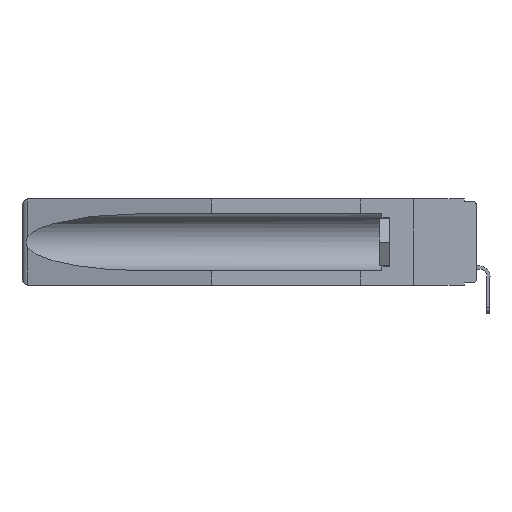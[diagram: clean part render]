
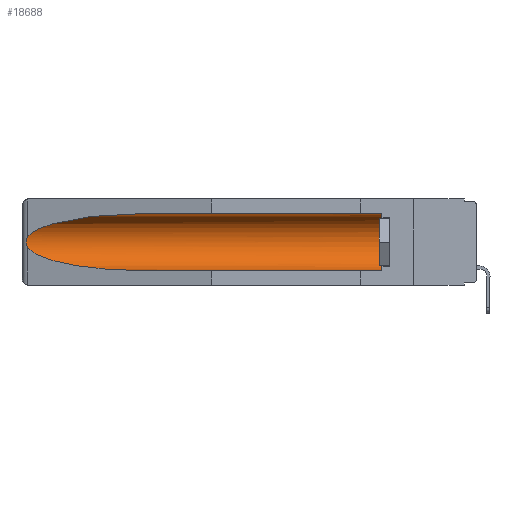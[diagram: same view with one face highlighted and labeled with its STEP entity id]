
A CAD part, left-side view. The second image highlights one B-rep face of the part: STEP entity #18688.
In plain terms, the highlighted cylindrical face has radius 2.857 mm (diameter 5.715 mm), a partial arc.
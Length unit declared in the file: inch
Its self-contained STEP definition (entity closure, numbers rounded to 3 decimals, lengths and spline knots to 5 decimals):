
#214 =( BOUNDED_CURVE ( )  B_SPLINE_CURVE ( 3, ( #3086, #10755, #3312, #23945 ),
 .UNSPECIFIED., .F., .F. ) 
 B_SPLINE_CURVE_WITH_KNOTS ( ( 4, 4 ),
 ( 0.1948, 1.5708 ),
 .UNSPECIFIED. ) 
 CURVE ( )  GEOMETRIC_REPRESENTATION_ITEM ( )  RATIONAL_B_SPLINE_CURVE ( ( 1., 0.848, 0.848, 1. ) ) 
 REPRESENTATION_ITEM ( '' )  );
#909 = CARTESIAN_POINT ( 'NONE',  ( 0.2675, 1.53308, -0.17534 ) ) ;
#1145 = CARTESIAN_POINT ( 'NONE',  ( 0.155, 0.126, -0.1715 ) ) ;
#1150 = CARTESIAN_POINT ( 'NONE',  ( 0.26597, 1.5296, -0.19026 ) ) ;
#1480 = ORIENTED_EDGE ( 'NONE', *, *, #16808, .T. ) ;
#1636 = CARTESIAN_POINT ( 'NONE',  ( 0.155, 1.07973, -0.284 ) ) ;
#1738 = B_SPLINE_CURVE_WITH_KNOTS ( 'NONE', 3,
 ( #10363, #10457, #4682, #23730, #18011, #909, #14199, #2793, #1150, #3044 ),
 .UNSPECIFIED., .F., .F.,
 ( 4, 2, 2, 2, 4 ),
 ( 0., 0.00029, 0.00058, 0.00087, 0.00117 ),
 .UNSPECIFIED. ) ;
#2286 = EDGE_CURVE ( 'NONE', #7174, #4447, #18360, .T. ) ;
#2654 = CARTESIAN_POINT ( 'NONE',  ( 0.155, -0.30754, -0.059 ) ) ;
#2793 = CARTESIAN_POINT ( 'NONE',  ( 0.26655, 1.53094, -0.18657 ) ) ;
#2854 = EDGE_CURVE ( 'NONE', #22755, #12830, #214, .T. ) ;
#3044 = CARTESIAN_POINT ( 'NONE',  ( 0.26537, 1.52718, -0.19328 ) ) ;
#3086 = CARTESIAN_POINT ( 'NONE',  ( 0.26537, 1.52718, -0.19328 ) ) ;
#3312 = CARTESIAN_POINT ( 'NONE',  ( 0.21114, 1.30732, -0.284 ) ) ;
#3334 = CARTESIAN_POINT ( 'NONE',  ( 0.155, -0.30754, -0.284 ) ) ;
#4349 = EDGE_LOOP ( 'NONE', ( #18473, #1480, #19409, #7672, #11660, #10160 ) ) ;
#4447 = VERTEX_POINT ( 'NONE', #12825 ) ;
#4682 = CARTESIAN_POINT ( 'NONE',  ( 0.26654, 1.53092, -0.15636 ) ) ;
#5478 = CARTESIAN_POINT ( 'NONE',  ( 0.155, 0.126, -0.284 ) ) ;
#6430 = DIRECTION ( 'NONE',  ( 0., 1., 0. ) ) ;
#6952 = DIRECTION ( 'NONE',  ( 0., 1., 0. ) ) ;
#7174 = VERTEX_POINT ( 'NONE', #5478 ) ;
#7672 = ORIENTED_EDGE ( 'NONE', *, *, #9293, .F. ) ;
#7790 = VECTOR ( 'NONE', #6430, 39.37008 ) ;
#8319 = CARTESIAN_POINT ( 'NONE',  ( 0.26537, 1.52718, -0.14972 ) ) ;
#8668 = DIRECTION ( 'NONE',  ( 0., 0., 1. ) ) ;
#9293 = EDGE_CURVE ( 'NONE', #7174, #12830, #16475, .T. ) ;
#10160 = ORIENTED_EDGE ( 'NONE', *, *, #16293, .T. ) ;
#10363 = CARTESIAN_POINT ( 'NONE',  ( 0.26537, 1.52718, -0.14972 ) ) ;
#10380 = VERTEX_POINT ( 'NONE', #24231 ) ;
#10457 = CARTESIAN_POINT ( 'NONE',  ( 0.26597, 1.52961, -0.15275 ) ) ;
#10755 = CARTESIAN_POINT ( 'NONE',  ( 0.25451, 1.48313, -0.24835 ) ) ;
#11124 = LINE ( 'NONE', #2654, #7790 ) ;
#11408 = VECTOR ( 'NONE', #16687, 39.37008 ) ;
#11660 = ORIENTED_EDGE ( 'NONE', *, *, #2286, .T. ) ;
#11787 = FACE_OUTER_BOUND ( 'NONE', #4349, .T. ) ;
#12029 = CARTESIAN_POINT ( 'NONE',  ( 0.21114, 1.30732, -0.059 ) ) ;
#12825 = CARTESIAN_POINT ( 'NONE',  ( 0.155, 0.126, -0.059 ) ) ;
#12830 = VERTEX_POINT ( 'NONE', #1636 ) ;
#14199 = CARTESIAN_POINT ( 'NONE',  ( 0.2673, 1.53269, -0.17917 ) ) ;
#15849 = CARTESIAN_POINT ( 'NONE',  ( 0.25451, 1.48313, -0.09465 ) ) ;
#16293 = EDGE_CURVE ( 'NONE', #4447, #10380, #11124, .T. ) ;
#16475 = LINE ( 'NONE', #3334, #11408 ) ;
#16501 = CARTESIAN_POINT ( 'NONE',  ( 0.155, -0.30754, -0.1715 ) ) ;
#16566 = CYLINDRICAL_SURFACE ( 'NONE', #23483, 0.1125 ) ;
#16687 = DIRECTION ( 'NONE',  ( 0., 1., 0. ) ) ;
#16808 = EDGE_CURVE ( 'NONE', #18762, #22755, #1738, .T. ) ;
#17666 = CARTESIAN_POINT ( 'NONE',  ( 0.155, 1.07973, -0.059 ) ) ;
#18011 = CARTESIAN_POINT ( 'NONE',  ( 0.2675, 1.53308, -0.16763 ) ) ;
#18360 = CIRCLE ( 'NONE', #19079, 0.1125 ) ;
#18473 = ORIENTED_EDGE ( 'NONE', *, *, #21146, .T. ) ;
#18688 = ADVANCED_FACE ( 'NONE', ( #11787 ), #16566, .F. ) ;
#18762 = VERTEX_POINT ( 'NONE', #21893 ) ;
#19079 = AXIS2_PLACEMENT_3D ( 'NONE', #1145, #20052, #8668 ) ;
#19409 = ORIENTED_EDGE ( 'NONE', *, *, #2854, .T. ) ;
#19999 =( BOUNDED_CURVE ( )  B_SPLINE_CURVE ( 3, ( #17666, #12029, #15849, #8319 ),
 .UNSPECIFIED., .F., .T. ) 
 B_SPLINE_CURVE_WITH_KNOTS ( ( 4, 4 ),
 ( 4.71239, 6.08839 ),
 .UNSPECIFIED. ) 
 CURVE ( )  GEOMETRIC_REPRESENTATION_ITEM ( )  RATIONAL_B_SPLINE_CURVE ( ( 1., 0.848, 0.848, 1. ) ) 
 REPRESENTATION_ITEM ( '' )  );
#20052 = DIRECTION ( 'NONE',  ( 0., -1., 0. ) ) ;
#21003 = CARTESIAN_POINT ( 'NONE',  ( 0.26537, 1.52718, -0.19328 ) ) ;
#21146 = EDGE_CURVE ( 'NONE', #10380, #18762, #19999, .T. ) ;
#21893 = CARTESIAN_POINT ( 'NONE',  ( 0.26537, 1.52718, -0.14972 ) ) ;
#22184 = DIRECTION ( 'NONE',  ( 0., 0., 1. ) ) ;
#22755 = VERTEX_POINT ( 'NONE', #21003 ) ;
#23483 = AXIS2_PLACEMENT_3D ( 'NONE', #16501, #6952, #22184 ) ;
#23730 = CARTESIAN_POINT ( 'NONE',  ( 0.2673, 1.5327, -0.16383 ) ) ;
#23945 = CARTESIAN_POINT ( 'NONE',  ( 0.155, 1.07973, -0.284 ) ) ;
#24231 = CARTESIAN_POINT ( 'NONE',  ( 0.155, 1.07973, -0.059 ) ) ;
